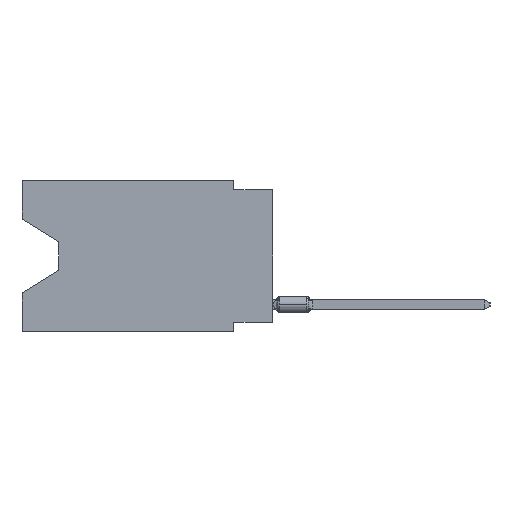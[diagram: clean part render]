
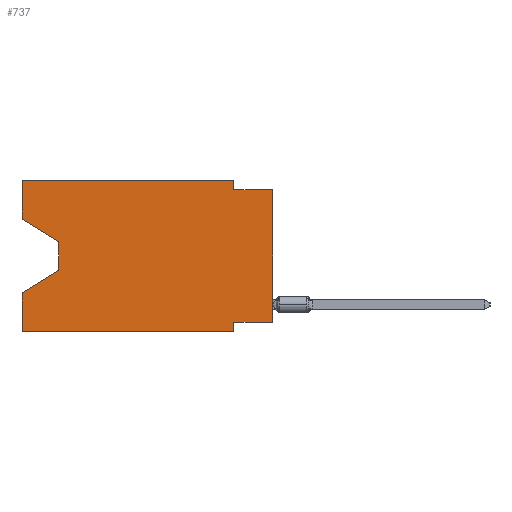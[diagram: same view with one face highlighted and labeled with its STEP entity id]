
A CAD part, left-side view. The second image highlights one B-rep face of the part: STEP entity #737.
In plain terms, the highlighted planar face has unit normal (-1, 0, 0).
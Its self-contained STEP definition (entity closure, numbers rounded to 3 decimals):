
#89 = CARTESIAN_POINT ( 'NONE',  ( 0., 0., 0. ) ) ;
#737 = ADVANCED_FACE ( 'NONE', ( #29871 ), #30819, .F. ) ;
#894 = LINE ( 'NONE', #6036, #4050 ) ;
#2669 = CARTESIAN_POINT ( 'NONE',  ( 0., 16.383, 0. ) ) ;
#3882 = CARTESIAN_POINT ( 'NONE',  ( 0., 16.383, -7.36 ) ) ;
#4050 = VECTOR ( 'NONE', #35578, 1000. ) ;
#4710 = ORIENTED_EDGE ( 'NONE', *, *, #60979, .F. ) ;
#4736 = VERTEX_POINT ( 'NONE', #17983 ) ;
#5708 = VECTOR ( 'NONE', #48775, 1000. ) ;
#6036 = CARTESIAN_POINT ( 'NONE',  ( 0., 0., -0.635 ) ) ;
#6532 = LINE ( 'NONE', #55324, #7194 ) ;
#7194 = VECTOR ( 'NONE', #25807, 1000. ) ;
#7197 = EDGE_CURVE ( 'NONE', #57851, #54557, #19962, .T. ) ;
#7294 = VERTEX_POINT ( 'NONE', #25754 ) ;
#7708 = CARTESIAN_POINT ( 'NONE',  ( 0., 2.54, -9.271 ) ) ;
#7963 = CARTESIAN_POINT ( 'NONE',  ( 0., 16.383, -2.546 ) ) ;
#9608 = LINE ( 'NONE', #18273, #5708 ) ;
#10308 = ORIENTED_EDGE ( 'NONE', *, *, #20384, .F. ) ;
#11914 = DIRECTION ( 'NONE',  ( 0., 1., 0. ) ) ;
#12869 = CARTESIAN_POINT ( 'NONE',  ( 0., 0., -0.635 ) ) ;
#13092 = CARTESIAN_POINT ( 'NONE',  ( 0., 16.383, 0. ) ) ;
#13659 = VERTEX_POINT ( 'NONE', #7708 ) ;
#14570 = VECTOR ( 'NONE', #37387, 1000. ) ;
#16008 = CARTESIAN_POINT ( 'NONE',  ( 0., 2.54, -0.635 ) ) ;
#16386 = ORIENTED_EDGE ( 'NONE', *, *, #7197, .T. ) ;
#16921 = LINE ( 'NONE', #32042, #25605 ) ;
#17699 = ORIENTED_EDGE ( 'NONE', *, *, #28607, .F. ) ;
#17983 = CARTESIAN_POINT ( 'NONE',  ( 0., 13.97, -5.893 ) ) ;
#18273 = CARTESIAN_POINT ( 'NONE',  ( 0., 13.97, -5.893 ) ) ;
#19216 = CARTESIAN_POINT ( 'NONE',  ( 0., 2.54, 0. ) ) ;
#19511 = AXIS2_PLACEMENT_3D ( 'NONE', #20208, #50043, #30185 ) ;
#19962 = LINE ( 'NONE', #24477, #48199 ) ;
#20208 = CARTESIAN_POINT ( 'NONE',  ( 0., 16.383, 0. ) ) ;
#20384 = EDGE_CURVE ( 'NONE', #63073, #45594, #894, .T. ) ;
#20544 = EDGE_CURVE ( 'NONE', #63208, #7294, #16921, .T. ) ;
#21058 = VERTEX_POINT ( 'NONE', #19216 ) ;
#21638 = DIRECTION ( 'NONE',  ( 0., -1., 0. ) ) ;
#24105 = VECTOR ( 'NONE', #54595, 1000. ) ;
#24477 = CARTESIAN_POINT ( 'NONE',  ( 0., 16.383, -9.906 ) ) ;
#24510 = LINE ( 'NONE', #89, #31018 ) ;
#25280 = EDGE_CURVE ( 'NONE', #30738, #45594, #24510, .T. ) ;
#25605 = VECTOR ( 'NONE', #47724, 1000. ) ;
#25754 = CARTESIAN_POINT ( 'NONE',  ( 0., 13.97, -4.013 ) ) ;
#25807 = DIRECTION ( 'NONE',  ( 0., 0., 1. ) ) ;
#27363 = LINE ( 'NONE', #38254, #24105 ) ;
#28607 = EDGE_CURVE ( 'NONE', #57851, #46674, #27363, .T. ) ;
#29871 = FACE_OUTER_BOUND ( 'NONE', #56354, .T. ) ;
#29910 = VECTOR ( 'NONE', #21638, 1000. ) ;
#30185 = DIRECTION ( 'NONE',  ( 0., 0., -1. ) ) ;
#30738 = VERTEX_POINT ( 'NONE', #55054 ) ;
#30819 = PLANE ( 'NONE',  #19511 ) ;
#30839 = VECTOR ( 'NONE', #61809, 1000. ) ;
#31018 = VECTOR ( 'NONE', #39580, 1000. ) ;
#32042 = CARTESIAN_POINT ( 'NONE',  ( 0., 16.383, -2.546 ) ) ;
#32327 = CARTESIAN_POINT ( 'NONE',  ( 0., 13.97, -4.013 ) ) ;
#32594 = EDGE_CURVE ( 'NONE', #7294, #4736, #47076, .T. ) ;
#33978 = CARTESIAN_POINT ( 'NONE',  ( 0., 16.383, -9.906 ) ) ;
#34125 = DIRECTION ( 'NONE',  ( 0., -1., 0. ) ) ;
#35578 = DIRECTION ( 'NONE',  ( 0., -1., 0. ) ) ;
#35757 = EDGE_CURVE ( 'NONE', #13659, #54557, #42255, .T. ) ;
#36089 = LINE ( 'NONE', #2669, #29910 ) ;
#36244 = EDGE_CURVE ( 'NONE', #63213, #21058, #36089, .T. ) ;
#36578 = EDGE_CURVE ( 'NONE', #30738, #13659, #55264, .T. ) ;
#36778 = CARTESIAN_POINT ( 'NONE',  ( 0., 2.54, -9.906 ) ) ;
#36953 = CARTESIAN_POINT ( 'NONE',  ( 0., 0., -9.271 ) ) ;
#37387 = DIRECTION ( 'NONE',  ( 0., 0., -1. ) ) ;
#37441 = DIRECTION ( 'NONE',  ( 0., 0., -1. ) ) ;
#38254 = CARTESIAN_POINT ( 'NONE',  ( 0., 16.383, 0. ) ) ;
#38354 = EDGE_CURVE ( 'NONE', #21058, #63073, #52467, .T. ) ;
#38510 = ORIENTED_EDGE ( 'NONE', *, *, #52692, .T. ) ;
#39580 = DIRECTION ( 'NONE',  ( 0., 0., 1. ) ) ;
#40470 = ORIENTED_EDGE ( 'NONE', *, *, #35757, .F. ) ;
#42234 = VECTOR ( 'NONE', #11914, 1000. ) ;
#42255 = LINE ( 'NONE', #36778, #30839 ) ;
#45492 = CARTESIAN_POINT ( 'NONE',  ( 0., 2.54, -9.906 ) ) ;
#45594 = VERTEX_POINT ( 'NONE', #12869 ) ;
#46674 = VERTEX_POINT ( 'NONE', #3882 ) ;
#47076 = LINE ( 'NONE', #32327, #57259 ) ;
#47643 = CARTESIAN_POINT ( 'NONE',  ( 0., 2.54, 0. ) ) ;
#47724 = DIRECTION ( 'NONE',  ( 0., -0.855, -0.519 ) ) ;
#48199 = VECTOR ( 'NONE', #34125, 1000. ) ;
#48775 = DIRECTION ( 'NONE',  ( 0., 0.855, -0.519 ) ) ;
#50043 = DIRECTION ( 'NONE',  ( 1., 0., 0. ) ) ;
#50256 = ORIENTED_EDGE ( 'NONE', *, *, #25280, .T. ) ;
#50671 = ORIENTED_EDGE ( 'NONE', *, *, #32594, .T. ) ;
#52467 = LINE ( 'NONE', #47643, #14570 ) ;
#52692 = EDGE_CURVE ( 'NONE', #4736, #46674, #9608, .T. ) ;
#54557 = VERTEX_POINT ( 'NONE', #45492 ) ;
#54595 = DIRECTION ( 'NONE',  ( 0., 0., 1. ) ) ;
#55054 = CARTESIAN_POINT ( 'NONE',  ( 0., 0., -9.271 ) ) ;
#55264 = LINE ( 'NONE', #36953, #42234 ) ;
#55324 = CARTESIAN_POINT ( 'NONE',  ( 0., 16.383, 0. ) ) ;
#56354 = EDGE_LOOP ( 'NONE', ( #58748, #50671, #38510, #17699, #16386, #40470, #62410, #50256, #10308, #60100, #63226, #4710 ) ) ;
#57259 = VECTOR ( 'NONE', #37441, 1000. ) ;
#57851 = VERTEX_POINT ( 'NONE', #33978 ) ;
#58748 = ORIENTED_EDGE ( 'NONE', *, *, #20544, .T. ) ;
#60100 = ORIENTED_EDGE ( 'NONE', *, *, #38354, .F. ) ;
#60979 = EDGE_CURVE ( 'NONE', #63208, #63213, #6532, .T. ) ;
#61809 = DIRECTION ( 'NONE',  ( 0., 0., -1. ) ) ;
#62410 = ORIENTED_EDGE ( 'NONE', *, *, #36578, .F. ) ;
#63073 = VERTEX_POINT ( 'NONE', #16008 ) ;
#63208 = VERTEX_POINT ( 'NONE', #7963 ) ;
#63213 = VERTEX_POINT ( 'NONE', #13092 ) ;
#63226 = ORIENTED_EDGE ( 'NONE', *, *, #36244, .F. ) ;
